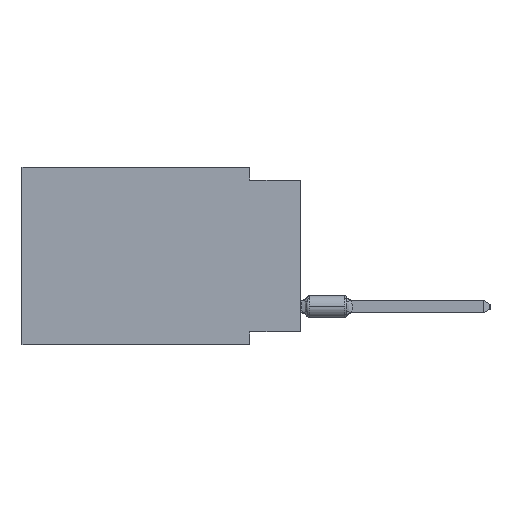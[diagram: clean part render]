
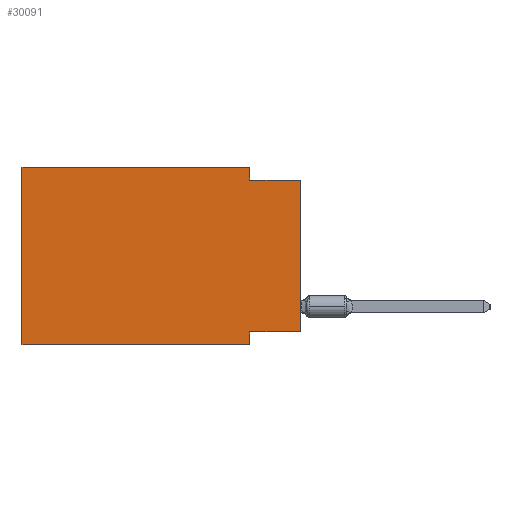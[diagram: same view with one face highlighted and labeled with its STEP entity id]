
A CAD part, left-side view. The second image highlights one B-rep face of the part: STEP entity #30091.
In plain terms, the highlighted planar face has unit normal (-1, 0, 0).
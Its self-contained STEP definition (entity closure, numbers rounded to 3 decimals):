
#896 = LINE ( 'NONE', #41591, #6544 ) ;
#917 = VERTEX_POINT ( 'NONE', #56996 ) ;
#1293 = EDGE_CURVE ( 'NONE', #22300, #15819, #25102, .T. ) ;
#4180 = VECTOR ( 'NONE', #32422, 1000. ) ;
#4787 = VERTEX_POINT ( 'NONE', #12372 ) ;
#5690 = VERTEX_POINT ( 'NONE', #40756 ) ;
#6337 = EDGE_CURVE ( 'NONE', #22300, #4787, #47145, .T. ) ;
#6544 = VECTOR ( 'NONE', #46608, 1000. ) ;
#11583 = ORIENTED_EDGE ( 'NONE', *, *, #17010, .F. ) ;
#12372 = CARTESIAN_POINT ( 'NONE',  ( 0., 13.97, 0. ) ) ;
#13331 = VECTOR ( 'NONE', #35297, 1000. ) ;
#14470 = ORIENTED_EDGE ( 'NONE', *, *, #40412, .F. ) ;
#14533 = EDGE_CURVE ( 'NONE', #17329, #24818, #896, .T. ) ;
#14757 = DIRECTION ( 'NONE',  ( 0., 1., 0. ) ) ;
#15170 = CARTESIAN_POINT ( 'NONE',  ( 0., 0., -0.635 ) ) ;
#15819 = VERTEX_POINT ( 'NONE', #33634 ) ;
#17010 = EDGE_CURVE ( 'NONE', #917, #15819, #31149, .T. ) ;
#17329 = VERTEX_POINT ( 'NONE', #22241 ) ;
#18604 = LINE ( 'NONE', #24212, #53129 ) ;
#22241 = CARTESIAN_POINT ( 'NONE',  ( 0., 2.54, -0.635 ) ) ;
#22300 = VERTEX_POINT ( 'NONE', #44262 ) ;
#22949 = VECTOR ( 'NONE', #37336, 1000. ) ;
#23000 = LINE ( 'NONE', #50099, #4180 ) ;
#24212 = CARTESIAN_POINT ( 'NONE',  ( 0., 0., -8.255 ) ) ;
#24818 = VERTEX_POINT ( 'NONE', #15170 ) ;
#25102 = LINE ( 'NONE', #43088, #53946 ) ;
#26308 = VERTEX_POINT ( 'NONE', #42932 ) ;
#27311 = CARTESIAN_POINT ( 'NONE',  ( 0., 2.54, -8.89 ) ) ;
#28289 = CARTESIAN_POINT ( 'NONE',  ( 0., 13.97, 0. ) ) ;
#28599 = ORIENTED_EDGE ( 'NONE', *, *, #51684, .F. ) ;
#28787 = LINE ( 'NONE', #45889, #22949 ) ;
#28968 = DIRECTION ( 'NONE',  ( 0., 0., -1. ) ) ;
#30091 = ADVANCED_FACE ( 'NONE', ( #50193 ), #36941, .F. ) ;
#30845 = DIRECTION ( 'NONE',  ( 0., -1., 0. ) ) ;
#31149 = LINE ( 'NONE', #27311, #13331 ) ;
#32422 = DIRECTION ( 'NONE',  ( 0., 0., -1. ) ) ;
#33634 = CARTESIAN_POINT ( 'NONE',  ( 0., 2.54, -8.89 ) ) ;
#34544 = EDGE_LOOP ( 'NONE', ( #53392, #45092, #14470, #41079, #37463, #51529, #11583, #28599 ) ) ;
#35297 = DIRECTION ( 'NONE',  ( 0., 0., -1. ) ) ;
#36941 = PLANE ( 'NONE',  #52429 ) ;
#37336 = DIRECTION ( 'NONE',  ( 0., 0., 1. ) ) ;
#37439 = DIRECTION ( 'NONE',  ( 0., 0., 1. ) ) ;
#37463 = ORIENTED_EDGE ( 'NONE', *, *, #6337, .F. ) ;
#37931 = VECTOR ( 'NONE', #30845, 1000. ) ;
#40412 = EDGE_CURVE ( 'NONE', #5690, #17329, #23000, .T. ) ;
#40756 = CARTESIAN_POINT ( 'NONE',  ( 0., 2.54, 0. ) ) ;
#41079 = ORIENTED_EDGE ( 'NONE', *, *, #49451, .F. ) ;
#41591 = CARTESIAN_POINT ( 'NONE',  ( 0., 0., -0.635 ) ) ;
#42932 = CARTESIAN_POINT ( 'NONE',  ( 0., 0., -8.255 ) ) ;
#43088 = CARTESIAN_POINT ( 'NONE',  ( 0., 13.97, -8.89 ) ) ;
#43545 = VECTOR ( 'NONE', #37439, 1000. ) ;
#44262 = CARTESIAN_POINT ( 'NONE',  ( 0., 13.97, -8.89 ) ) ;
#44695 = CARTESIAN_POINT ( 'NONE',  ( 0., 13.97, 0. ) ) ;
#45092 = ORIENTED_EDGE ( 'NONE', *, *, #14533, .F. ) ;
#45889 = CARTESIAN_POINT ( 'NONE',  ( 0., 0., 0. ) ) ;
#46608 = DIRECTION ( 'NONE',  ( 0., -1., 0. ) ) ;
#46664 = DIRECTION ( 'NONE',  ( 1., 0., 0. ) ) ;
#47145 = LINE ( 'NONE', #28289, #43545 ) ;
#49098 = LINE ( 'NONE', #44695, #37931 ) ;
#49451 = EDGE_CURVE ( 'NONE', #4787, #5690, #49098, .T. ) ;
#50099 = CARTESIAN_POINT ( 'NONE',  ( 0., 2.54, 0. ) ) ;
#50193 = FACE_OUTER_BOUND ( 'NONE', #34544, .T. ) ;
#51074 = CARTESIAN_POINT ( 'NONE',  ( 0., 13.97, 0. ) ) ;
#51529 = ORIENTED_EDGE ( 'NONE', *, *, #1293, .T. ) ;
#51684 = EDGE_CURVE ( 'NONE', #26308, #917, #18604, .T. ) ;
#52429 = AXIS2_PLACEMENT_3D ( 'NONE', #51074, #46664, #28968 ) ;
#53129 = VECTOR ( 'NONE', #14757, 1000. ) ;
#53392 = ORIENTED_EDGE ( 'NONE', *, *, #54958, .T. ) ;
#53946 = VECTOR ( 'NONE', #56627, 1000. ) ;
#54958 = EDGE_CURVE ( 'NONE', #26308, #24818, #28787, .T. ) ;
#56627 = DIRECTION ( 'NONE',  ( 0., -1., 0. ) ) ;
#56996 = CARTESIAN_POINT ( 'NONE',  ( 0., 2.54, -8.255 ) ) ;
